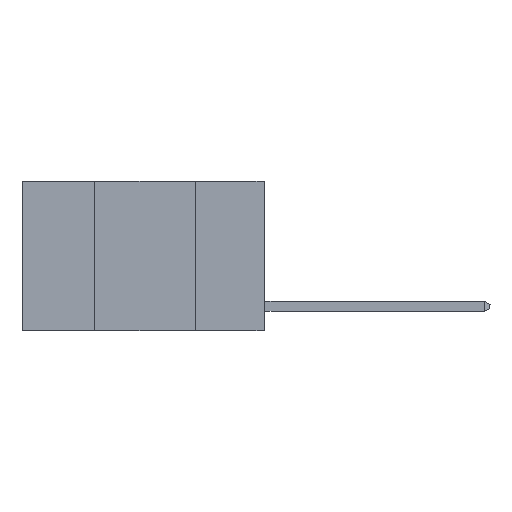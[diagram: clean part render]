
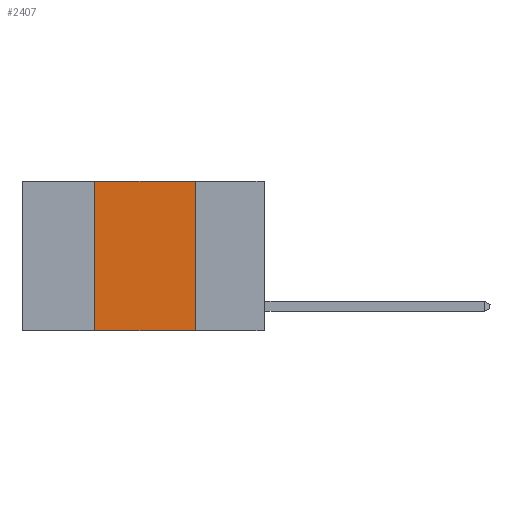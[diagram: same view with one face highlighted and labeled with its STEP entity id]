
A CAD part, left-side view. The second image highlights one B-rep face of the part: STEP entity #2407.
In plain terms, the highlighted planar face has unit normal (-1, 0, 0).
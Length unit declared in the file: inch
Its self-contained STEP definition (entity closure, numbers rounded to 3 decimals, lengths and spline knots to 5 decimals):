
#437 = AXIS2_PLACEMENT_3D ( 'NONE', #25423, #23884, #23826 ) ;
#627 = CARTESIAN_POINT ( 'NONE',  ( 0., 0.42, 0. ) ) ;
#884 = CARTESIAN_POINT ( 'NONE',  ( 0., 0.17, 0. ) ) ;
#1292 = EDGE_CURVE ( 'NONE', #14698, #20227, #16174, .T. ) ;
#1325 = ORIENTED_EDGE ( 'NONE', *, *, #1292, .F. ) ;
#1382 = VECTOR ( 'NONE', #2226, 39.37008 ) ;
#1422 = EDGE_LOOP ( 'NONE', ( #6163, #21937, #1325, #12080 ) ) ;
#2226 = DIRECTION ( 'NONE',  ( 0., 0., 1. ) ) ;
#2371 = EDGE_CURVE ( 'NONE', #20227, #7894, #20466, .T. ) ;
#2407 = ADVANCED_FACE ( 'NONE', ( #19258 ), #4717, .F. ) ;
#2434 = CARTESIAN_POINT ( 'NONE',  ( 0., 0.42, 0. ) ) ;
#4072 = EDGE_CURVE ( 'NONE', #7894, #10169, #24362, .T. ) ;
#4642 = VECTOR ( 'NONE', #18996, 39.37008 ) ;
#4717 = PLANE ( 'NONE',  #437 ) ;
#5050 = DIRECTION ( 'NONE',  ( 0., 0., -1. ) ) ;
#6163 = ORIENTED_EDGE ( 'NONE', *, *, #4072, .F. ) ;
#7894 = VERTEX_POINT ( 'NONE', #18177 ) ;
#10169 = VERTEX_POINT ( 'NONE', #24494 ) ;
#11344 = DIRECTION ( 'NONE',  ( 0., -1., 0. ) ) ;
#12080 = ORIENTED_EDGE ( 'NONE', *, *, #25721, .T. ) ;
#13307 = CARTESIAN_POINT ( 'NONE',  ( 0., 0.6, -0.37 ) ) ;
#14698 = VERTEX_POINT ( 'NONE', #16731 ) ;
#16174 = LINE ( 'NONE', #2434, #1382 ) ;
#16731 = CARTESIAN_POINT ( 'NONE',  ( 0., 0.42, -0.37 ) ) ;
#17373 = VECTOR ( 'NONE', #11344, 39.37008 ) ;
#18177 = CARTESIAN_POINT ( 'NONE',  ( 0., 0.17, 0. ) ) ;
#18996 = DIRECTION ( 'NONE',  ( 0., -1., 0. ) ) ;
#19258 = FACE_OUTER_BOUND ( 'NONE', #1422, .T. ) ;
#20227 = VERTEX_POINT ( 'NONE', #627 ) ;
#20466 = LINE ( 'NONE', #20545, #4642 ) ;
#20545 = CARTESIAN_POINT ( 'NONE',  ( 0., 0.6, 0. ) ) ;
#21937 = ORIENTED_EDGE ( 'NONE', *, *, #2371, .F. ) ;
#22560 = LINE ( 'NONE', #13307, #17373 ) ;
#23168 = VECTOR ( 'NONE', #5050, 39.37008 ) ;
#23826 = DIRECTION ( 'NONE',  ( 0., 0., -1. ) ) ;
#23884 = DIRECTION ( 'NONE',  ( 1., 0., 0. ) ) ;
#24362 = LINE ( 'NONE', #884, #23168 ) ;
#24494 = CARTESIAN_POINT ( 'NONE',  ( 0., 0.17, -0.37 ) ) ;
#25423 = CARTESIAN_POINT ( 'NONE',  ( 0., 0.6, 0. ) ) ;
#25721 = EDGE_CURVE ( 'NONE', #14698, #10169, #22560, .T. ) ;
